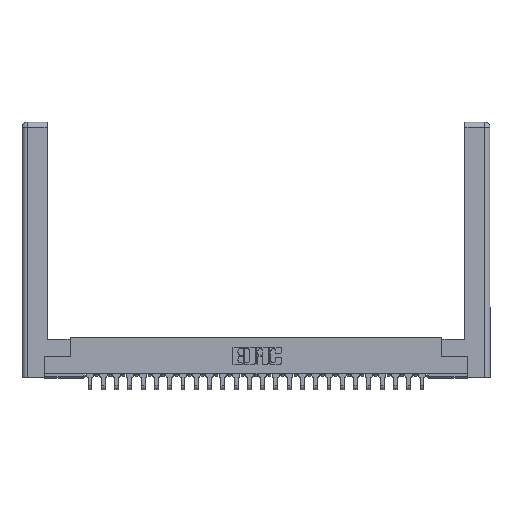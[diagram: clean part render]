
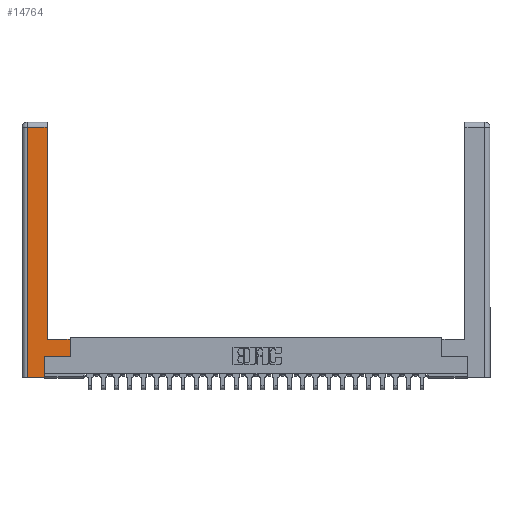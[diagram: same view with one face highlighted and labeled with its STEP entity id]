
A CAD part, top view. The second image highlights one B-rep face of the part: STEP entity #14764.
In plain terms, the highlighted planar face has unit normal (0, 0, 1).
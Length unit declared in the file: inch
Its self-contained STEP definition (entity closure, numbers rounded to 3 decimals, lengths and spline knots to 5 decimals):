
#12 = VECTOR ( 'NONE', #7394, 39.37008 ) ;
#90 = LINE ( 'NONE', #17785, #13087 ) ;
#119 = LINE ( 'NONE', #18622, #19922 ) ;
#573 = VECTOR ( 'NONE', #2167, 39.37008 ) ;
#1593 = CARTESIAN_POINT ( 'NONE',  ( 0.295, 0.45, 0. ) ) ;
#1858 = ORIENTED_EDGE ( 'NONE', *, *, #16654, .T. ) ;
#1977 = EDGE_CURVE ( 'NONE', #3949, #15301, #13971, .T. ) ;
#2167 = DIRECTION ( 'NONE',  ( -1., 0., 0. ) ) ;
#3135 = CARTESIAN_POINT ( 'NONE',  ( 0.565, 0.45, 0. ) ) ;
#3531 = DIRECTION ( 'NONE',  ( 1., 0., 0. ) ) ;
#3949 = VERTEX_POINT ( 'NONE', #1593 ) ;
#4145 = ORIENTED_EDGE ( 'NONE', *, *, #25330, .T. ) ;
#4351 = CARTESIAN_POINT ( 'NONE',  ( 0.0615, 2.94, 0. ) ) ;
#4528 = CARTESIAN_POINT ( 'NONE',  ( 0.265, 0.245, 0. ) ) ;
#4624 = ORIENTED_EDGE ( 'NONE', *, *, #9463, .T. ) ;
#5850 = CARTESIAN_POINT ( 'NONE',  ( 0.295, 2.94, 0. ) ) ;
#7038 = VECTOR ( 'NONE', #9664, 39.37008 ) ;
#7074 = AXIS2_PLACEMENT_3D ( 'NONE', #14561, #24608, #20457 ) ;
#7207 = ORIENTED_EDGE ( 'NONE', *, *, #8984, .T. ) ;
#7394 = DIRECTION ( 'NONE',  ( 0., 1., 0. ) ) ;
#7749 = EDGE_CURVE ( 'NONE', #25204, #12274, #22754, .T. ) ;
#8984 = EDGE_CURVE ( 'NONE', #13044, #25204, #119, .T. ) ;
#9360 = DIRECTION ( 'NONE',  ( -1., 0., 0. ) ) ;
#9463 = EDGE_CURVE ( 'NONE', #12940, #3949, #90, .T. ) ;
#9664 = DIRECTION ( 'NONE',  ( 0., 1., 0. ) ) ;
#9987 = ORIENTED_EDGE ( 'NONE', *, *, #1977, .T. ) ;
#11308 = LINE ( 'NONE', #4351, #573 ) ;
#12274 = VERTEX_POINT ( 'NONE', #17684 ) ;
#12302 = CARTESIAN_POINT ( 'NONE',  ( 0.0615, 2.94, 0. ) ) ;
#12563 = EDGE_CURVE ( 'NONE', #15301, #13044, #11308, .T. ) ;
#12940 = VERTEX_POINT ( 'NONE', #22207 ) ;
#13044 = VERTEX_POINT ( 'NONE', #12302 ) ;
#13087 = VECTOR ( 'NONE', #9360, 39.37008 ) ;
#13530 = CARTESIAN_POINT ( 'NONE',  ( 0.265, 0.245, 0. ) ) ;
#13971 = LINE ( 'NONE', #18414, #23468 ) ;
#14561 = CARTESIAN_POINT ( 'NONE',  ( 0., 0., 0. ) ) ;
#14764 = ADVANCED_FACE ( 'NONE', ( #21597 ), #15840, .F. ) ;
#15301 = VERTEX_POINT ( 'NONE', #5850 ) ;
#15796 = LINE ( 'NONE', #22612, #25953 ) ;
#15840 = PLANE ( 'NONE',  #7074 ) ;
#16110 = LINE ( 'NONE', #13530, #7038 ) ;
#16131 = ORIENTED_EDGE ( 'NONE', *, *, #7749, .T. ) ;
#16308 = ORIENTED_EDGE ( 'NONE', *, *, #22182, .T. ) ;
#16654 = EDGE_CURVE ( 'NONE', #16866, #24426, #15796, .T. ) ;
#16866 = VERTEX_POINT ( 'NONE', #4528 ) ;
#17684 = CARTESIAN_POINT ( 'NONE',  ( 0.265, 0., 0. ) ) ;
#17785 = CARTESIAN_POINT ( 'NONE',  ( 0.295, 0.45, 0. ) ) ;
#18122 = CARTESIAN_POINT ( 'NONE',  ( 0.265, 0., 0. ) ) ;
#18414 = CARTESIAN_POINT ( 'NONE',  ( 0.295, 3., 0. ) ) ;
#18622 = CARTESIAN_POINT ( 'NONE',  ( 0.0615, 0., 0. ) ) ;
#19271 = ORIENTED_EDGE ( 'NONE', *, *, #12563, .T. ) ;
#19813 = LINE ( 'NONE', #3135, #12 ) ;
#19922 = VECTOR ( 'NONE', #22819, 39.37008 ) ;
#20233 = DIRECTION ( 'NONE',  ( 0., 1., 0. ) ) ;
#20457 = DIRECTION ( 'NONE',  ( -1., 0., 0. ) ) ;
#21364 = CARTESIAN_POINT ( 'NONE',  ( 0.0615, 0., 0. ) ) ;
#21597 = FACE_OUTER_BOUND ( 'NONE', #25125, .T. ) ;
#22182 = EDGE_CURVE ( 'NONE', #24426, #12940, #19813, .T. ) ;
#22207 = CARTESIAN_POINT ( 'NONE',  ( 0.565, 0.45, 0. ) ) ;
#22612 = CARTESIAN_POINT ( 'NONE',  ( 0.565, 0.245, 0. ) ) ;
#22754 = LINE ( 'NONE', #18122, #23435 ) ;
#22819 = DIRECTION ( 'NONE',  ( 0., -1., 0. ) ) ;
#23295 = CARTESIAN_POINT ( 'NONE',  ( 0.565, 0.245, 0. ) ) ;
#23435 = VECTOR ( 'NONE', #26660, 39.37008 ) ;
#23468 = VECTOR ( 'NONE', #20233, 39.37008 ) ;
#24426 = VERTEX_POINT ( 'NONE', #23295 ) ;
#24608 = DIRECTION ( 'NONE',  ( 0., 0., -1. ) ) ;
#25125 = EDGE_LOOP ( 'NONE', ( #9987, #19271, #7207, #16131, #4145, #1858, #16308, #4624 ) ) ;
#25204 = VERTEX_POINT ( 'NONE', #21364 ) ;
#25330 = EDGE_CURVE ( 'NONE', #12274, #16866, #16110, .T. ) ;
#25953 = VECTOR ( 'NONE', #3531, 39.37008 ) ;
#26660 = DIRECTION ( 'NONE',  ( 1., 0., 0. ) ) ;
